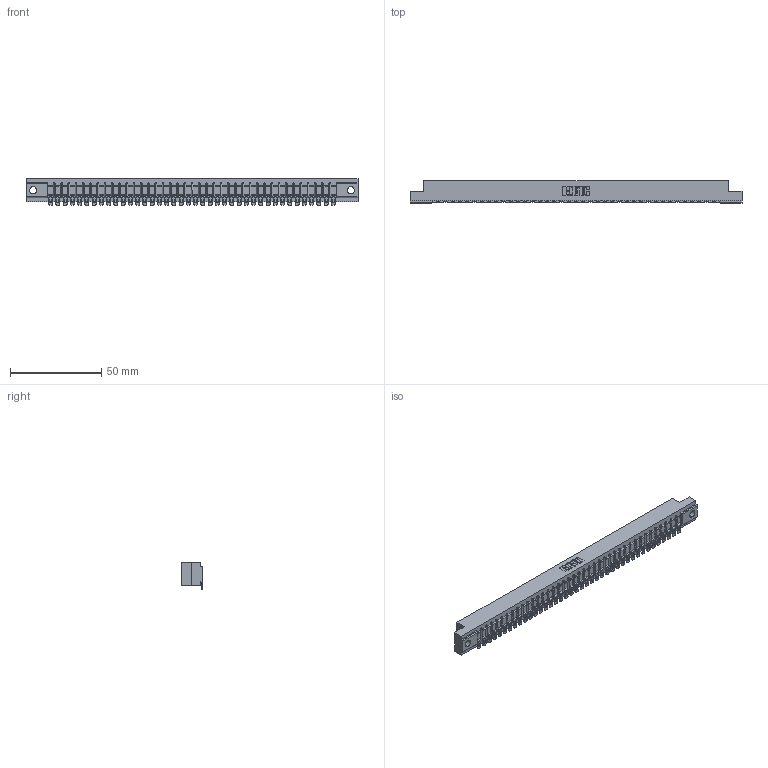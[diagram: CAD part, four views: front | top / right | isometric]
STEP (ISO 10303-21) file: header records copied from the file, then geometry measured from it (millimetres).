
FILE_DESCRIPTION (( 'STEP AP203' ), '1' );
FILE_NAME ('357-040-554-104.STEP', '2019-09-17T09:15:47', ( '' ), ( '' ), 'SwSTEP 2.0', 'SolidWorks 2016', '' );
FILE_SCHEMA (( 'CONFIG_CONTROL_DESIGN' ));
Length unit declared in the file: inch
Products named in the file (3): 307 Part_.156 Dia Mounting Holes; 307-290-002_554; 357-040-554-104
Assembly tree (41 placements, depth 2):
  357-040-554-104
    307 Part_.156 Dia Mounting Holes
    307-290-002_554  x40
Bounding box: 181.51 x 12.01 x 14.52 mm (x, y, z)
Volume: 19317.2 mm3; surface area: 24234.7 mm2
Topology: 41 solids, 41 shells, 3413 faces, 10479 edges, 6874 vertices
Faces by surface type: plane 1924, cylinder 1407, sphere 82
Entity records: 35921 total; most frequent: CARTESIAN_POINT 6064, ORIENTED_EDGE 6052, DIRECTION 5890, EDGE_CURVE 3026, LINE 2318, VECTOR 2318, VERTEX_POINT 1960, AXIS2_PLACEMENT_3D 1786
